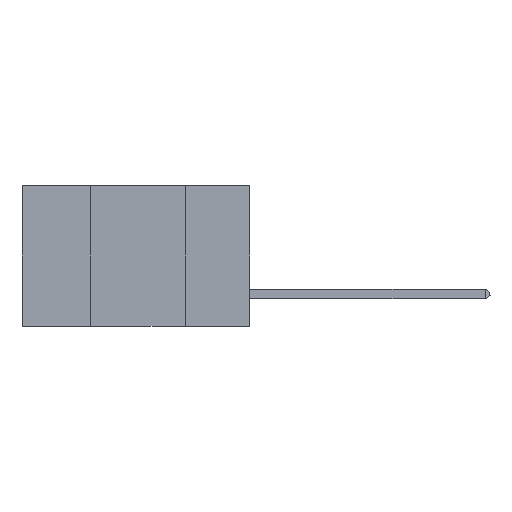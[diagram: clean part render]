
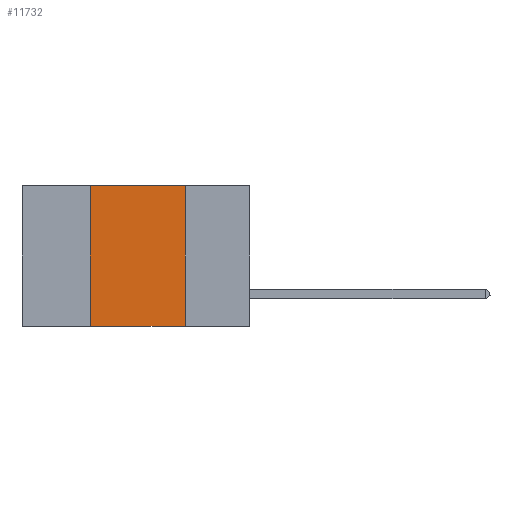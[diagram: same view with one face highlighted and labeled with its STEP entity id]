
A CAD part, left-side view. The second image highlights one B-rep face of the part: STEP entity #11732.
In plain terms, the highlighted planar face has unit normal (-1, 0, 0).
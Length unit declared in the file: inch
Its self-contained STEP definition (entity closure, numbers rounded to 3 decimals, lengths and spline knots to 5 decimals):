
#88 = CARTESIAN_POINT ( 'NONE',  ( 0., 0.6, 0. ) ) ;
#1234 = DIRECTION ( 'NONE',  ( 0., 0., -1. ) ) ;
#1355 = EDGE_CURVE ( 'NONE', #10063, #4287, #7417, .T. ) ;
#2194 = ORIENTED_EDGE ( 'NONE', *, *, #1355, .T. ) ;
#2407 = DIRECTION ( 'NONE',  ( 0., 0., 1. ) ) ;
#2507 = DIRECTION ( 'NONE',  ( 0., -1., 0. ) ) ;
#2768 = LINE ( 'NONE', #88, #4465 ) ;
#2876 = AXIS2_PLACEMENT_3D ( 'NONE', #6514, #14990, #14766 ) ;
#3203 = VECTOR ( 'NONE', #2407, 39.37008 ) ;
#3622 = CARTESIAN_POINT ( 'NONE',  ( 0., 0.17, 0. ) ) ;
#4287 = VERTEX_POINT ( 'NONE', #7335 ) ;
#4465 = VECTOR ( 'NONE', #9851, 39.37008 ) ;
#5149 = ORIENTED_EDGE ( 'NONE', *, *, #12640, .F. ) ;
#5183 = EDGE_CURVE ( 'NONE', #9377, #11709, #2768, .T. ) ;
#6514 = CARTESIAN_POINT ( 'NONE',  ( 0., 0.6, 0. ) ) ;
#7335 = CARTESIAN_POINT ( 'NONE',  ( 0., 0.17, -0.37 ) ) ;
#7417 = LINE ( 'NONE', #13289, #10175 ) ;
#7418 = CARTESIAN_POINT ( 'NONE',  ( 0., 0.42, -0.37 ) ) ;
#8086 = LINE ( 'NONE', #14426, #3203 ) ;
#8720 = ORIENTED_EDGE ( 'NONE', *, *, #5183, .F. ) ;
#8828 = VECTOR ( 'NONE', #1234, 39.37008 ) ;
#8892 = EDGE_LOOP ( 'NONE', ( #5149, #8720, #13976, #2194 ) ) ;
#9377 = VERTEX_POINT ( 'NONE', #11422 ) ;
#9851 = DIRECTION ( 'NONE',  ( 0., -1., 0. ) ) ;
#10063 = VERTEX_POINT ( 'NONE', #7418 ) ;
#10175 = VECTOR ( 'NONE', #2507, 39.37008 ) ;
#10761 = CARTESIAN_POINT ( 'NONE',  ( 0., 0.17, 0. ) ) ;
#11422 = CARTESIAN_POINT ( 'NONE',  ( 0., 0.42, 0. ) ) ;
#11709 = VERTEX_POINT ( 'NONE', #3622 ) ;
#11732 = ADVANCED_FACE ( 'NONE', ( #12454 ), #13526, .F. ) ;
#12454 = FACE_OUTER_BOUND ( 'NONE', #8892, .T. ) ;
#12640 = EDGE_CURVE ( 'NONE', #11709, #4287, #13958, .T. ) ;
#12778 = EDGE_CURVE ( 'NONE', #10063, #9377, #8086, .T. ) ;
#13289 = CARTESIAN_POINT ( 'NONE',  ( 0., 0.6, -0.37 ) ) ;
#13526 = PLANE ( 'NONE',  #2876 ) ;
#13958 = LINE ( 'NONE', #10761, #8828 ) ;
#13976 = ORIENTED_EDGE ( 'NONE', *, *, #12778, .F. ) ;
#14426 = CARTESIAN_POINT ( 'NONE',  ( 0., 0.42, 0. ) ) ;
#14766 = DIRECTION ( 'NONE',  ( 0., 0., -1. ) ) ;
#14990 = DIRECTION ( 'NONE',  ( 1., 0., 0. ) ) ;
